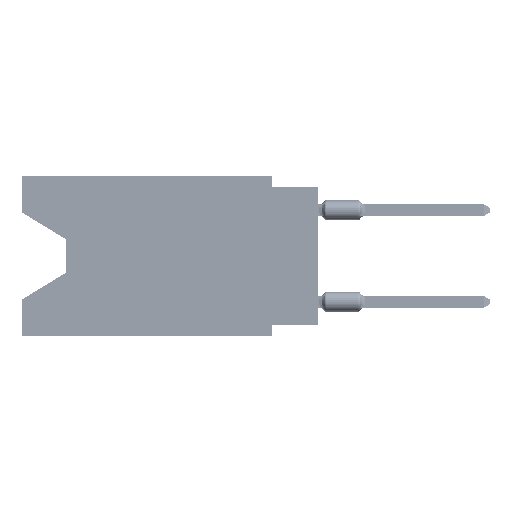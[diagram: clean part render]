
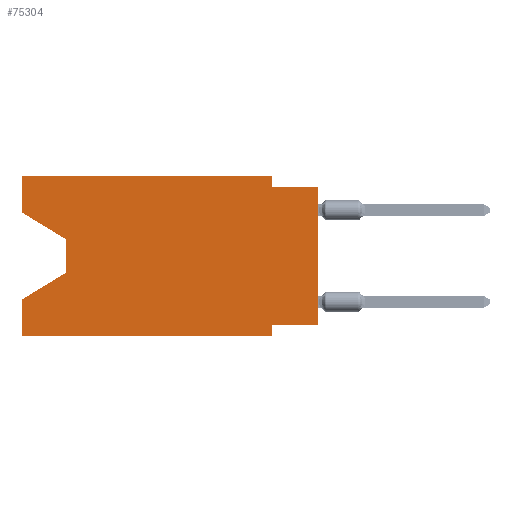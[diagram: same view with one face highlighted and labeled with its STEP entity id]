
A CAD part, left-side view. The second image highlights one B-rep face of the part: STEP entity #75304.
In plain terms, the highlighted planar face has unit normal (-1, 0, 0).
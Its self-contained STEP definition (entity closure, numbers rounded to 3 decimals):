
#769 = EDGE_LOOP ( 'NONE', ( #75641, #40871, #49073, #14381, #62740, #3004, #7977, #60847, #66774, #46511, #24997, #47364 ) ) ;
#906 = DIRECTION ( 'NONE',  ( 0., 0., 1. ) ) ;
#1609 = CARTESIAN_POINT ( 'NONE',  ( 0., 16.383, -6.852 ) ) ;
#2965 = CARTESIAN_POINT ( 'NONE',  ( 0., 16.383, -8.89 ) ) ;
#3004 = ORIENTED_EDGE ( 'NONE', *, *, #19805, .F. ) ;
#3180 = FACE_OUTER_BOUND ( 'NONE', #769, .T. ) ;
#5605 = CARTESIAN_POINT ( 'NONE',  ( 0., 0., -8.255 ) ) ;
#7977 = ORIENTED_EDGE ( 'NONE', *, *, #61872, .F. ) ;
#8249 = VERTEX_POINT ( 'NONE', #5605 ) ;
#8418 = EDGE_CURVE ( 'NONE', #54315, #11453, #20300, .T. ) ;
#9692 = LINE ( 'NONE', #35336, #65981 ) ;
#10682 = LINE ( 'NONE', #56086, #50249 ) ;
#11453 = VERTEX_POINT ( 'NONE', #1609 ) ;
#11710 = VERTEX_POINT ( 'NONE', #57035 ) ;
#11954 = CARTESIAN_POINT ( 'NONE',  ( 0., 16.383, 0. ) ) ;
#13436 = CARTESIAN_POINT ( 'NONE',  ( 0., 13.97, -5.385 ) ) ;
#14381 = ORIENTED_EDGE ( 'NONE', *, *, #27347, .F. ) ;
#14581 = CARTESIAN_POINT ( 'NONE',  ( 0., 13.97, -3.505 ) ) ;
#14839 = EDGE_CURVE ( 'NONE', #70737, #82053, #34992, .T. ) ;
#16065 = CARTESIAN_POINT ( 'NONE',  ( 0., 2.54, -8.255 ) ) ;
#16300 = VECTOR ( 'NONE', #33258, 1000. ) ;
#18921 = VECTOR ( 'NONE', #18963, 1000. ) ;
#18963 = DIRECTION ( 'NONE',  ( 0., 1., 0. ) ) ;
#19481 = DIRECTION ( 'NONE',  ( 0., 0., -1. ) ) ;
#19805 = EDGE_CURVE ( 'NONE', #35470, #61657, #46712, .T. ) ;
#20300 = LINE ( 'NONE', #45936, #58136 ) ;
#21079 = LINE ( 'NONE', #11954, #64007 ) ;
#23635 = LINE ( 'NONE', #81636, #52323 ) ;
#24058 = CARTESIAN_POINT ( 'NONE',  ( 0., 16.383, -2.038 ) ) ;
#24997 = ORIENTED_EDGE ( 'NONE', *, *, #14839, .F. ) ;
#26138 = CARTESIAN_POINT ( 'NONE',  ( 0., 16.383, -8.89 ) ) ;
#27240 = CARTESIAN_POINT ( 'NONE',  ( 0., 2.54, -0.635 ) ) ;
#27347 = EDGE_CURVE ( 'NONE', #81418, #11453, #21079, .T. ) ;
#28005 = DIRECTION ( 'NONE',  ( 0., 0., -1. ) ) ;
#28823 = PLANE ( 'NONE',  #65587 ) ;
#28931 = CARTESIAN_POINT ( 'NONE',  ( 0., 2.54, 0. ) ) ;
#32664 = CARTESIAN_POINT ( 'NONE',  ( 0., 0., -0.635 ) ) ;
#33258 = DIRECTION ( 'NONE',  ( 0., 0., -1. ) ) ;
#33547 = CARTESIAN_POINT ( 'NONE',  ( 0., 16.383, 0. ) ) ;
#34992 = LINE ( 'NONE', #74900, #68216 ) ;
#35336 = CARTESIAN_POINT ( 'NONE',  ( 0., 16.383, 0. ) ) ;
#35470 = VERTEX_POINT ( 'NONE', #16065 ) ;
#36185 = VERTEX_POINT ( 'NONE', #27240 ) ;
#36665 = DIRECTION ( 'NONE',  ( 0., -1., 0. ) ) ;
#36706 = EDGE_CURVE ( 'NONE', #36185, #65894, #23635, .T. ) ;
#38314 = LINE ( 'NONE', #51764, #18921 ) ;
#38414 = EDGE_CURVE ( 'NONE', #74854, #70737, #9692, .T. ) ;
#39381 = DIRECTION ( 'NONE',  ( 0., 0., -1. ) ) ;
#40871 = ORIENTED_EDGE ( 'NONE', *, *, #65999, .T. ) ;
#40924 = CARTESIAN_POINT ( 'NONE',  ( 0., 0., 0. ) ) ;
#45348 = EDGE_CURVE ( 'NONE', #8249, #65894, #79182, .T. ) ;
#45528 = CARTESIAN_POINT ( 'NONE',  ( 0., 2.54, 0. ) ) ;
#45871 = CARTESIAN_POINT ( 'NONE',  ( 0., 2.54, -8.89 ) ) ;
#45936 = CARTESIAN_POINT ( 'NONE',  ( 0., 13.97, -5.385 ) ) ;
#46050 = VECTOR ( 'NONE', #66454, 1000. ) ;
#46511 = ORIENTED_EDGE ( 'NONE', *, *, #78532, .F. ) ;
#46712 = LINE ( 'NONE', #45871, #16300 ) ;
#47364 = ORIENTED_EDGE ( 'NONE', *, *, #38414, .F. ) ;
#49073 = ORIENTED_EDGE ( 'NONE', *, *, #8418, .T. ) ;
#50249 = VECTOR ( 'NONE', #74576, 1000. ) ;
#50601 = LINE ( 'NONE', #45528, #82087 ) ;
#51764 = CARTESIAN_POINT ( 'NONE',  ( 0., 0., -8.255 ) ) ;
#52323 = VECTOR ( 'NONE', #36665, 1000. ) ;
#53116 = CARTESIAN_POINT ( 'NONE',  ( 0., 2.54, -8.89 ) ) ;
#54315 = VERTEX_POINT ( 'NONE', #13436 ) ;
#55469 = VECTOR ( 'NONE', #39381, 1000. ) ;
#56086 = CARTESIAN_POINT ( 'NONE',  ( 0., 16.383, -2.038 ) ) ;
#57035 = CARTESIAN_POINT ( 'NONE',  ( 0., 13.97, -3.505 ) ) ;
#58136 = VECTOR ( 'NONE', #71571, 1000. ) ;
#59976 = LINE ( 'NONE', #14581, #55469 ) ;
#60847 = ORIENTED_EDGE ( 'NONE', *, *, #45348, .T. ) ;
#60988 = DIRECTION ( 'NONE',  ( 0., 0., 1. ) ) ;
#61657 = VERTEX_POINT ( 'NONE', #53116 ) ;
#61872 = EDGE_CURVE ( 'NONE', #8249, #35470, #38314, .T. ) ;
#62740 = ORIENTED_EDGE ( 'NONE', *, *, #63915, .T. ) ;
#63915 = EDGE_CURVE ( 'NONE', #81418, #61657, #78244, .T. ) ;
#64007 = VECTOR ( 'NONE', #906, 1000. ) ;
#65587 = AXIS2_PLACEMENT_3D ( 'NONE', #73392, #78886, #28005 ) ;
#65894 = VERTEX_POINT ( 'NONE', #32664 ) ;
#65981 = VECTOR ( 'NONE', #60988, 1000. ) ;
#65999 = EDGE_CURVE ( 'NONE', #11710, #54315, #59976, .T. ) ;
#66454 = DIRECTION ( 'NONE',  ( 0., -1., 0. ) ) ;
#66563 = DIRECTION ( 'NONE',  ( 0., 0., 1. ) ) ;
#66774 = ORIENTED_EDGE ( 'NONE', *, *, #36706, .F. ) ;
#67340 = DIRECTION ( 'NONE',  ( 0., -1., 0. ) ) ;
#68216 = VECTOR ( 'NONE', #67340, 1000. ) ;
#69259 = VECTOR ( 'NONE', #66563, 1000. ) ;
#70737 = VERTEX_POINT ( 'NONE', #33547 ) ;
#71571 = DIRECTION ( 'NONE',  ( 0., 0.855, -0.519 ) ) ;
#73392 = CARTESIAN_POINT ( 'NONE',  ( 0., 16.383, 0. ) ) ;
#74576 = DIRECTION ( 'NONE',  ( 0., -0.855, -0.519 ) ) ;
#74854 = VERTEX_POINT ( 'NONE', #24058 ) ;
#74900 = CARTESIAN_POINT ( 'NONE',  ( 0., 16.383, 0. ) ) ;
#75304 = ADVANCED_FACE ( 'NONE', ( #3180 ), #28823, .F. ) ;
#75641 = ORIENTED_EDGE ( 'NONE', *, *, #82270, .T. ) ;
#78244 = LINE ( 'NONE', #2965, #46050 ) ;
#78532 = EDGE_CURVE ( 'NONE', #82053, #36185, #50601, .T. ) ;
#78886 = DIRECTION ( 'NONE',  ( 1., 0., 0. ) ) ;
#79182 = LINE ( 'NONE', #40924, #69259 ) ;
#81418 = VERTEX_POINT ( 'NONE', #26138 ) ;
#81636 = CARTESIAN_POINT ( 'NONE',  ( 0., 0., -0.635 ) ) ;
#82053 = VERTEX_POINT ( 'NONE', #28931 ) ;
#82087 = VECTOR ( 'NONE', #19481, 1000. ) ;
#82270 = EDGE_CURVE ( 'NONE', #74854, #11710, #10682, .T. ) ;
